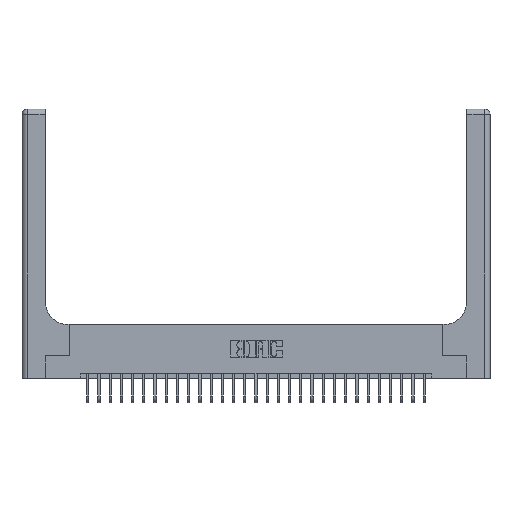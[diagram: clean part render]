
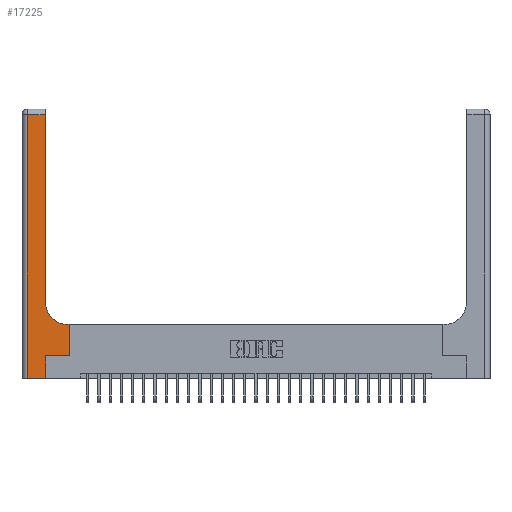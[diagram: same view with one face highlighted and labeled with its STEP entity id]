
A CAD part, top view. The second image highlights one B-rep face of the part: STEP entity #17225.
In plain terms, the highlighted planar face has unit normal (0, 0, 1).
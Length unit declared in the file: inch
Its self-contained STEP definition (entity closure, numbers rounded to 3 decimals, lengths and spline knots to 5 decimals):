
#509 = CARTESIAN_POINT ( 'NONE',  ( 0.06, 2.94, 0.37 ) ) ;
#667 = EDGE_LOOP ( 'NONE', ( #22986, #17990, #4030, #18386, #14957, #20342, #7074, #12231, #21782 ) ) ;
#696 = LINE ( 'NONE', #27684, #26041 ) ;
#1069 = VERTEX_POINT ( 'NONE', #4619 ) ;
#1154 = DIRECTION ( 'NONE',  ( -1., 0., 0. ) ) ;
#2741 = EDGE_CURVE ( 'NONE', #20555, #21932, #18050, .T. ) ;
#2935 = LINE ( 'NONE', #9576, #5782 ) ;
#3004 = DIRECTION ( 'NONE',  ( 1., 0., 0. ) ) ;
#4030 = ORIENTED_EDGE ( 'NONE', *, *, #10455, .T. ) ;
#4140 = VERTEX_POINT ( 'NONE', #26755 ) ;
#4163 = VERTEX_POINT ( 'NONE', #13924 ) ;
#4619 = CARTESIAN_POINT ( 'NONE',  ( 0.528, 0.6, 0.37 ) ) ;
#5202 = EDGE_CURVE ( 'NONE', #4163, #22533, #14903, .T. ) ;
#5313 = VECTOR ( 'NONE', #3004, 39.37008 ) ;
#5782 = VECTOR ( 'NONE', #18589, 39.37008 ) ;
#6257 = VECTOR ( 'NONE', #8908, 39.37008 ) ;
#6463 = DIRECTION ( 'NONE',  ( 1., 0., 0. ) ) ;
#6780 = VERTEX_POINT ( 'NONE', #28295 ) ;
#6972 = VECTOR ( 'NONE', #20736, 39.37008 ) ;
#7074 = ORIENTED_EDGE ( 'NONE', *, *, #7258, .T. ) ;
#7258 = EDGE_CURVE ( 'NONE', #21932, #1069, #696, .T. ) ;
#7452 = DIRECTION ( 'NONE',  ( 0., 1., 0. ) ) ;
#7871 = CARTESIAN_POINT ( 'NONE',  ( 0.06, 3., 0.37 ) ) ;
#7877 = AXIS2_PLACEMENT_3D ( 'NONE', #13698, #26819, #6463 ) ;
#7906 = CARTESIAN_POINT ( 'NONE',  ( 0., 3., 0.37 ) ) ;
#7980 = CARTESIAN_POINT ( 'NONE',  ( 0.265, 0.25, 0.37 ) ) ;
#8038 = DIRECTION ( 'NONE',  ( 0., 0., -1. ) ) ;
#8349 = CIRCLE ( 'NONE', #7877, 0.25 ) ;
#8653 = DIRECTION ( 'NONE',  ( -1., 0., 0. ) ) ;
#8661 = VECTOR ( 'NONE', #21825, 39.37008 ) ;
#8908 = DIRECTION ( 'NONE',  ( -1., 0., 0. ) ) ;
#9261 = VECTOR ( 'NONE', #24526, 39.37008 ) ;
#9576 = CARTESIAN_POINT ( 'NONE',  ( 0.265, 0., 0.37 ) ) ;
#10455 = EDGE_CURVE ( 'NONE', #20348, #4140, #16460, .T. ) ;
#11020 = CARTESIAN_POINT ( 'NONE',  ( 0., 2.94, 0.37 ) ) ;
#11570 = LINE ( 'NONE', #26900, #6257 ) ;
#11697 = CARTESIAN_POINT ( 'NONE',  ( 0.265, 0.25, 0.37 ) ) ;
#12231 = ORIENTED_EDGE ( 'NONE', *, *, #25698, .T. ) ;
#13698 = CARTESIAN_POINT ( 'NONE',  ( 0.51, 0.85, 0.37 ) ) ;
#13924 = CARTESIAN_POINT ( 'NONE',  ( 0.26, 0.85, 0.37 ) ) ;
#14086 = LINE ( 'NONE', #16442, #5313 ) ;
#14903 = LINE ( 'NONE', #23898, #8661 ) ;
#14957 = ORIENTED_EDGE ( 'NONE', *, *, #23322, .T. ) ;
#15807 = AXIS2_PLACEMENT_3D ( 'NONE', #7906, #8038, #1154 ) ;
#15892 = CARTESIAN_POINT ( 'NONE',  ( 0.528, 0.25, 0.37 ) ) ;
#16442 = CARTESIAN_POINT ( 'NONE',  ( 0., 0., 0.37 ) ) ;
#16460 = LINE ( 'NONE', #7871, #6972 ) ;
#17067 = PLANE ( 'NONE',  #15807 ) ;
#17225 = ADVANCED_FACE ( 'NONE', ( #25627 ), #17067, .F. ) ;
#17990 = ORIENTED_EDGE ( 'NONE', *, *, #21807, .T. ) ;
#18050 = LINE ( 'NONE', #11697, #9261 ) ;
#18148 = EDGE_CURVE ( 'NONE', #6780, #4163, #8349, .T. ) ;
#18386 = ORIENTED_EDGE ( 'NONE', *, *, #25872, .T. ) ;
#18589 = DIRECTION ( 'NONE',  ( 0., 1., 0. ) ) ;
#18918 = VECTOR ( 'NONE', #8653, 39.37008 ) ;
#19871 = LINE ( 'NONE', #11020, #18918 ) ;
#20342 = ORIENTED_EDGE ( 'NONE', *, *, #2741, .T. ) ;
#20348 = VERTEX_POINT ( 'NONE', #509 ) ;
#20555 = VERTEX_POINT ( 'NONE', #7980 ) ;
#20736 = DIRECTION ( 'NONE',  ( 0., -1., 0. ) ) ;
#21782 = ORIENTED_EDGE ( 'NONE', *, *, #18148, .T. ) ;
#21807 = EDGE_CURVE ( 'NONE', #22533, #20348, #19871, .T. ) ;
#21825 = DIRECTION ( 'NONE',  ( 0., 1., 0. ) ) ;
#21932 = VERTEX_POINT ( 'NONE', #15892 ) ;
#22343 = CARTESIAN_POINT ( 'NONE',  ( 0.265, 0., 0.37 ) ) ;
#22533 = VERTEX_POINT ( 'NONE', #23065 ) ;
#22986 = ORIENTED_EDGE ( 'NONE', *, *, #5202, .T. ) ;
#23065 = CARTESIAN_POINT ( 'NONE',  ( 0.26, 2.94, 0.37 ) ) ;
#23322 = EDGE_CURVE ( 'NONE', #23599, #20555, #2935, .T. ) ;
#23599 = VERTEX_POINT ( 'NONE', #22343 ) ;
#23898 = CARTESIAN_POINT ( 'NONE',  ( 0.26, 3., 0.37 ) ) ;
#24526 = DIRECTION ( 'NONE',  ( 1., 0., 0. ) ) ;
#25627 = FACE_OUTER_BOUND ( 'NONE', #667, .T. ) ;
#25698 = EDGE_CURVE ( 'NONE', #1069, #6780, #11570, .T. ) ;
#25872 = EDGE_CURVE ( 'NONE', #4140, #23599, #14086, .T. ) ;
#26041 = VECTOR ( 'NONE', #7452, 39.37008 ) ;
#26755 = CARTESIAN_POINT ( 'NONE',  ( 0.06, 0., 0.37 ) ) ;
#26819 = DIRECTION ( 'NONE',  ( 0., 0., -1. ) ) ;
#26900 = CARTESIAN_POINT ( 'NONE',  ( 0.26, 0.6, 0.37 ) ) ;
#27684 = CARTESIAN_POINT ( 'NONE',  ( 0.528, 0.25, 0.37 ) ) ;
#28295 = CARTESIAN_POINT ( 'NONE',  ( 0.51, 0.6, 0.37 ) ) ;
